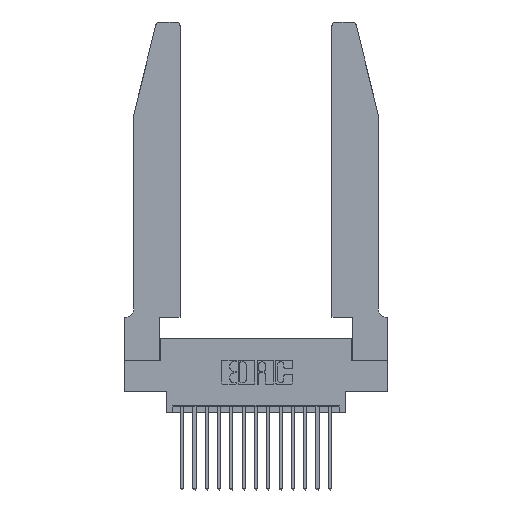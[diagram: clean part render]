
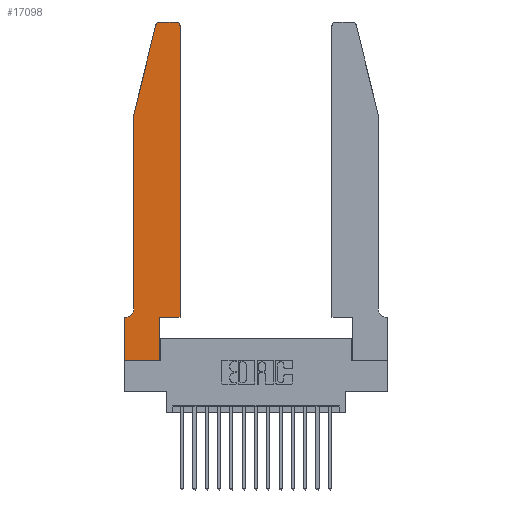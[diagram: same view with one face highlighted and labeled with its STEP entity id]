
A CAD part, top view. The second image highlights one B-rep face of the part: STEP entity #17098.
In plain terms, the highlighted planar face has unit normal (0, 0, 1).
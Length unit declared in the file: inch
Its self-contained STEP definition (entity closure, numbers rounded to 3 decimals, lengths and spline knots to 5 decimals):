
#294 = CARTESIAN_POINT ( 'NONE',  ( 0., 0., 0.37 ) ) ;
#339 = VECTOR ( 'NONE', #1569, 39.37008 ) ;
#414 = CARTESIAN_POINT ( 'NONE',  ( 0.0755, 0.42, 0.37 ) ) ;
#950 = ORIENTED_EDGE ( 'NONE', *, *, #3617, .T. ) ;
#987 = CARTESIAN_POINT ( 'NONE',  ( 0.2865, 0., 0.37 ) ) ;
#1311 = DIRECTION ( 'NONE',  ( 1., 0., 0. ) ) ;
#1569 = DIRECTION ( 'NONE',  ( 0., 1., 0. ) ) ;
#1813 = AXIS2_PLACEMENT_3D ( 'NONE', #14063, #18386, #9797 ) ;
#1819 = CIRCLE ( 'NONE', #7774, 0.07 ) ;
#2079 = CARTESIAN_POINT ( 'NONE',  ( 0.0755, 2., 0.37 ) ) ;
#2275 = CARTESIAN_POINT ( 'NONE',  ( 0.2865, 0.35, 0.37 ) ) ;
#2606 = VERTEX_POINT ( 'NONE', #2870 ) ;
#2742 = CARTESIAN_POINT ( 'NONE',  ( 0.0755, 0.35, 0.37 ) ) ;
#2870 = CARTESIAN_POINT ( 'NONE',  ( 0.284, 2.75, 0.37 ) ) ;
#3079 = VERTEX_POINT ( 'NONE', #9217 ) ;
#3428 = ORIENTED_EDGE ( 'NONE', *, *, #4007, .T. ) ;
#3534 = LINE ( 'NONE', #13923, #10880 ) ;
#3617 = EDGE_CURVE ( 'NONE', #11409, #6615, #14823, .T. ) ;
#4007 = EDGE_CURVE ( 'NONE', #12637, #14977, #6251, .T. ) ;
#4068 = ORIENTED_EDGE ( 'NONE', *, *, #11780, .T. ) ;
#4158 = DIRECTION ( 'NONE',  ( -1., 0., 0. ) ) ;
#4229 = VECTOR ( 'NONE', #5141, 39.37008 ) ;
#4473 = CARTESIAN_POINT ( 'NONE',  ( 0., 0., 0.37 ) ) ;
#4635 = CARTESIAN_POINT ( 'NONE',  ( 0.4205, 2.72, 0.37 ) ) ;
#4827 = VECTOR ( 'NONE', #14461, 39.37008 ) ;
#5141 = DIRECTION ( 'NONE',  ( -0.239, -0.971, 0. ) ) ;
#5389 = CARTESIAN_POINT ( 'NONE',  ( 0.0755, 2., 0.37 ) ) ;
#5541 = EDGE_CURVE ( 'NONE', #2606, #3079, #7782, .T. ) ;
#5704 = VERTEX_POINT ( 'NONE', #9391 ) ;
#5745 = CARTESIAN_POINT ( 'NONE',  ( 0., 0., 0.37 ) ) ;
#5841 = ORIENTED_EDGE ( 'NONE', *, *, #15277, .T. ) ;
#6146 = DIRECTION ( 'NONE',  ( 1., 0., 0. ) ) ;
#6187 = DIRECTION ( 'NONE',  ( 0., 1., 0. ) ) ;
#6251 = LINE ( 'NONE', #18391, #13004 ) ;
#6337 = EDGE_CURVE ( 'NONE', #8594, #11409, #3534, .T. ) ;
#6416 = VECTOR ( 'NONE', #7593, 39.37008 ) ;
#6544 = ORIENTED_EDGE ( 'NONE', *, *, #16876, .T. ) ;
#6615 = VERTEX_POINT ( 'NONE', #16011 ) ;
#6745 = DIRECTION ( 'NONE',  ( 1., 0., 0. ) ) ;
#6863 = ORIENTED_EDGE ( 'NONE', *, *, #8415, .T. ) ;
#6906 = CARTESIAN_POINT ( 'NONE',  ( 0.0055, 0.42, 0.37 ) ) ;
#7011 = VERTEX_POINT ( 'NONE', #5745 ) ;
#7593 = DIRECTION ( 'NONE',  ( 0., -1., 0. ) ) ;
#7613 = VECTOR ( 'NONE', #6187, 39.37008 ) ;
#7774 = AXIS2_PLACEMENT_3D ( 'NONE', #6906, #16990, #8370 ) ;
#7782 = CIRCLE ( 'NONE', #15809, 0.03 ) ;
#8184 = LINE ( 'NONE', #2079, #4229 ) ;
#8370 = DIRECTION ( 'NONE',  ( -1., 0., 0. ) ) ;
#8405 = LINE ( 'NONE', #17709, #339 ) ;
#8415 = EDGE_CURVE ( 'NONE', #7011, #15890, #12642, .T. ) ;
#8594 = VERTEX_POINT ( 'NONE', #2275 ) ;
#8999 = VERTEX_POINT ( 'NONE', #9128 ) ;
#9086 = ORIENTED_EDGE ( 'NONE', *, *, #18381, .T. ) ;
#9128 = CARTESIAN_POINT ( 'NONE',  ( 0., 0.35, 0.37 ) ) ;
#9217 = CARTESIAN_POINT ( 'NONE',  ( 0.25487, 2.72718, 0.37 ) ) ;
#9224 = LINE ( 'NONE', #2742, #4827 ) ;
#9327 = ORIENTED_EDGE ( 'NONE', *, *, #12937, .T. ) ;
#9391 = CARTESIAN_POINT ( 'NONE',  ( 0.0055, 0.35, 0.37 ) ) ;
#9431 = CARTESIAN_POINT ( 'NONE',  ( 0.4505, 0.35, 0.37 ) ) ;
#9689 = VECTOR ( 'NONE', #4158, 39.37008 ) ;
#9739 = VECTOR ( 'NONE', #16501, 39.37008 ) ;
#9797 = DIRECTION ( 'NONE',  ( 1., 0., 0. ) ) ;
#10252 = DIRECTION ( 'NONE',  ( 0., 0., 1. ) ) ;
#10711 = LINE ( 'NONE', #4473, #6416 ) ;
#10880 = VECTOR ( 'NONE', #6745, 39.37008 ) ;
#11007 = EDGE_LOOP ( 'NONE', ( #18778, #18846, #15895, #3428, #9086, #5841, #6544, #6863, #9327, #13036, #950, #4068 ) ) ;
#11229 = DIRECTION ( 'NONE',  ( 0., -1., 0. ) ) ;
#11322 = CIRCLE ( 'NONE', #13807, 0.03 ) ;
#11409 = VERTEX_POINT ( 'NONE', #9431 ) ;
#11438 = CARTESIAN_POINT ( 'NONE',  ( 0.2605, 2.75, 0.37 ) ) ;
#11780 = EDGE_CURVE ( 'NONE', #6615, #16317, #11322, .T. ) ;
#11994 = EDGE_CURVE ( 'NONE', #3079, #12637, #8184, .T. ) ;
#12637 = VERTEX_POINT ( 'NONE', #5389 ) ;
#12642 = LINE ( 'NONE', #294, #9739 ) ;
#12937 = EDGE_CURVE ( 'NONE', #15890, #8594, #8405, .T. ) ;
#13004 = VECTOR ( 'NONE', #11229, 39.37008 ) ;
#13036 = ORIENTED_EDGE ( 'NONE', *, *, #6337, .T. ) ;
#13807 = AXIS2_PLACEMENT_3D ( 'NONE', #4635, #14806, #6146 ) ;
#13923 = CARTESIAN_POINT ( 'NONE',  ( 0.4505, 0.35, 0.37 ) ) ;
#13944 = LINE ( 'NONE', #11438, #9689 ) ;
#14063 = CARTESIAN_POINT ( 'NONE',  ( 0., 0.35, 0.37 ) ) ;
#14461 = DIRECTION ( 'NONE',  ( -1., 0., 0. ) ) ;
#14704 = EDGE_CURVE ( 'NONE', #16317, #2606, #13944, .T. ) ;
#14806 = DIRECTION ( 'NONE',  ( 0., 0., 1. ) ) ;
#14823 = LINE ( 'NONE', #14855, #7613 ) ;
#14855 = CARTESIAN_POINT ( 'NONE',  ( 0.4505, 0.35, 0.37 ) ) ;
#14977 = VERTEX_POINT ( 'NONE', #414 ) ;
#15242 = CARTESIAN_POINT ( 'NONE',  ( 0.4205, 2.75, 0.37 ) ) ;
#15277 = EDGE_CURVE ( 'NONE', #5704, #8999, #9224, .T. ) ;
#15809 = AXIS2_PLACEMENT_3D ( 'NONE', #18821, #10252, #1311 ) ;
#15890 = VERTEX_POINT ( 'NONE', #987 ) ;
#15895 = ORIENTED_EDGE ( 'NONE', *, *, #11994, .T. ) ;
#16011 = CARTESIAN_POINT ( 'NONE',  ( 0.4505, 2.72, 0.37 ) ) ;
#16317 = VERTEX_POINT ( 'NONE', #15242 ) ;
#16501 = DIRECTION ( 'NONE',  ( 1., 0., 0. ) ) ;
#16876 = EDGE_CURVE ( 'NONE', #8999, #7011, #10711, .T. ) ;
#16969 = PLANE ( 'NONE',  #1813 ) ;
#16990 = DIRECTION ( 'NONE',  ( 0., 0., -1. ) ) ;
#17098 = ADVANCED_FACE ( 'NONE', ( #17686 ), #16969, .T. ) ;
#17686 = FACE_OUTER_BOUND ( 'NONE', #11007, .T. ) ;
#17709 = CARTESIAN_POINT ( 'NONE',  ( 0.2865, 0.35, 0.37 ) ) ;
#18381 = EDGE_CURVE ( 'NONE', #14977, #5704, #1819, .T. ) ;
#18386 = DIRECTION ( 'NONE',  ( 0., 0., 1. ) ) ;
#18391 = CARTESIAN_POINT ( 'NONE',  ( 0.0755, 2., 0.37 ) ) ;
#18778 = ORIENTED_EDGE ( 'NONE', *, *, #14704, .T. ) ;
#18821 = CARTESIAN_POINT ( 'NONE',  ( 0.284, 2.72, 0.37 ) ) ;
#18846 = ORIENTED_EDGE ( 'NONE', *, *, #5541, .T. ) ;
